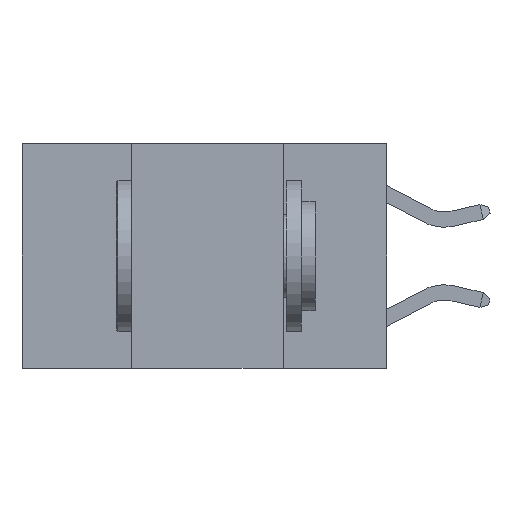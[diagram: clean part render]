
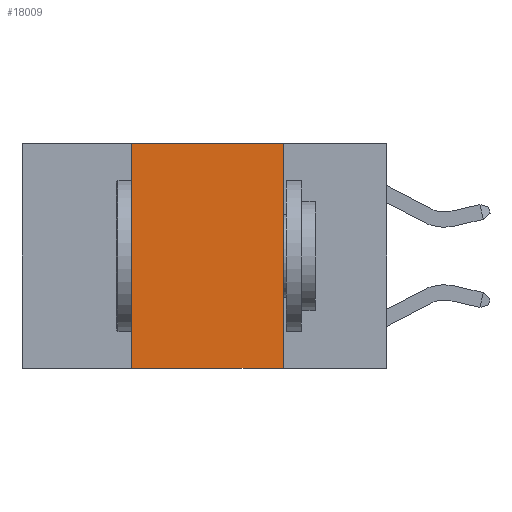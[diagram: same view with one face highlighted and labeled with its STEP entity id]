
A CAD part, left-side view. The second image highlights one B-rep face of the part: STEP entity #18009.
In plain terms, the highlighted planar face has unit normal (-1, 0, 0).
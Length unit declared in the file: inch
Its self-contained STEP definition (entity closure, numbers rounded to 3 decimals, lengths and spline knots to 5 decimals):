
#1273 = VECTOR ( 'NONE', #16100, 39.37008 ) ;
#2145 = LINE ( 'NONE', #8156, #1273 ) ;
#2405 = FACE_OUTER_BOUND ( 'NONE', #14594, .T. ) ;
#2715 = VERTEX_POINT ( 'NONE', #16006 ) ;
#3589 = VECTOR ( 'NONE', #22177, 39.37008 ) ;
#4101 = PLANE ( 'NONE',  #24421 ) ;
#4498 = CARTESIAN_POINT ( 'NONE',  ( 0., 0.6, 0. ) ) ;
#6476 = CARTESIAN_POINT ( 'NONE',  ( 0., 0.6, 0. ) ) ;
#6517 = EDGE_CURVE ( 'NONE', #2715, #14132, #16771, .T. ) ;
#8156 = CARTESIAN_POINT ( 'NONE',  ( 0., 0.17, 0. ) ) ;
#8207 = VERTEX_POINT ( 'NONE', #24721 ) ;
#8853 = CARTESIAN_POINT ( 'NONE',  ( 0., 0.17, 0. ) ) ;
#8947 = DIRECTION ( 'NONE',  ( 0., -1., 0. ) ) ;
#9085 = ORIENTED_EDGE ( 'NONE', *, *, #10935, .F. ) ;
#10792 = VERTEX_POINT ( 'NONE', #8853 ) ;
#10935 = EDGE_CURVE ( 'NONE', #10792, #14132, #2145, .T. ) ;
#10962 = EDGE_CURVE ( 'NONE', #8207, #10792, #14541, .T. ) ;
#14132 = VERTEX_POINT ( 'NONE', #22103 ) ;
#14211 = LINE ( 'NONE', #15899, #3589 ) ;
#14541 = LINE ( 'NONE', #4498, #15850 ) ;
#14594 = EDGE_LOOP ( 'NONE', ( #9085, #22590, #17142, #23357 ) ) ;
#14844 = CARTESIAN_POINT ( 'NONE',  ( 0., 0.6, -0.37 ) ) ;
#15850 = VECTOR ( 'NONE', #18423, 39.37008 ) ;
#15899 = CARTESIAN_POINT ( 'NONE',  ( 0., 0.42, 0. ) ) ;
#16006 = CARTESIAN_POINT ( 'NONE',  ( 0., 0.42, -0.37 ) ) ;
#16100 = DIRECTION ( 'NONE',  ( 0., 0., -1. ) ) ;
#16430 = EDGE_CURVE ( 'NONE', #2715, #8207, #14211, .T. ) ;
#16771 = LINE ( 'NONE', #14844, #20622 ) ;
#17142 = ORIENTED_EDGE ( 'NONE', *, *, #16430, .F. ) ;
#18009 = ADVANCED_FACE ( 'NONE', ( #2405 ), #4101, .F. ) ;
#18049 = DIRECTION ( 'NONE',  ( 1., 0., 0. ) ) ;
#18423 = DIRECTION ( 'NONE',  ( 0., -1., 0. ) ) ;
#20261 = DIRECTION ( 'NONE',  ( 0., 0., -1. ) ) ;
#20622 = VECTOR ( 'NONE', #8947, 39.37008 ) ;
#22103 = CARTESIAN_POINT ( 'NONE',  ( 0., 0.17, -0.37 ) ) ;
#22177 = DIRECTION ( 'NONE',  ( 0., 0., 1. ) ) ;
#22590 = ORIENTED_EDGE ( 'NONE', *, *, #10962, .F. ) ;
#23357 = ORIENTED_EDGE ( 'NONE', *, *, #6517, .T. ) ;
#24421 = AXIS2_PLACEMENT_3D ( 'NONE', #6476, #18049, #20261 ) ;
#24721 = CARTESIAN_POINT ( 'NONE',  ( 0., 0.42, 0. ) ) ;
